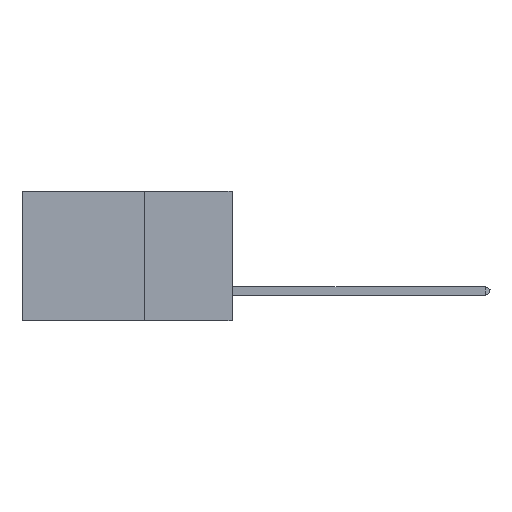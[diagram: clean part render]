
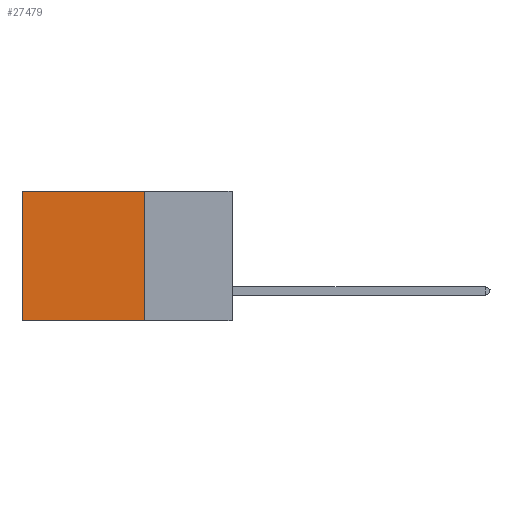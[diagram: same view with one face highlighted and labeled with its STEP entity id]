
A CAD part, left-side view. The second image highlights one B-rep face of the part: STEP entity #27479.
In plain terms, the highlighted planar face has unit normal (-1, 0, 0).
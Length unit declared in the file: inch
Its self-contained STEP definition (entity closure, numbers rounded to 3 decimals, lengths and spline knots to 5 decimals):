
#812 = PLANE ( 'NONE',  #20107 ) ;
#837 = CARTESIAN_POINT ( 'NONE',  ( 0.2875, 0.6, 0. ) ) ;
#2189 = EDGE_CURVE ( 'NONE', #25283, #23253, #4001, .T. ) ;
#4001 = LINE ( 'NONE', #10953, #29038 ) ;
#4308 = ORIENTED_EDGE ( 'NONE', *, *, #27179, .T. ) ;
#5876 = CARTESIAN_POINT ( 'NONE',  ( 0.2875, 0.25, 0. ) ) ;
#6701 = VERTEX_POINT ( 'NONE', #24163 ) ;
#7078 = LINE ( 'NONE', #837, #10500 ) ;
#7468 = EDGE_CURVE ( 'NONE', #6701, #9893, #19962, .T. ) ;
#7688 = VECTOR ( 'NONE', #10622, 39.37008 ) ;
#8294 = ORIENTED_EDGE ( 'NONE', *, *, #2189, .F. ) ;
#8321 = EDGE_CURVE ( 'NONE', #6701, #25283, #19513, .T. ) ;
#8379 = DIRECTION ( 'NONE',  ( 0., 1., 0. ) ) ;
#8865 = ORIENTED_EDGE ( 'NONE', *, *, #7468, .T. ) ;
#9514 = EDGE_LOOP ( 'NONE', ( #4308, #8294, #21635, #8865 ) ) ;
#9893 = VERTEX_POINT ( 'NONE', #20082 ) ;
#10471 = VECTOR ( 'NONE', #8379, 39.37008 ) ;
#10500 = VECTOR ( 'NONE', #17503, 39.37008 ) ;
#10622 = DIRECTION ( 'NONE',  ( 0., 0., -1. ) ) ;
#10794 = DIRECTION ( 'NONE',  ( 0., 0., -1. ) ) ;
#10953 = CARTESIAN_POINT ( 'NONE',  ( 0.2875, 0.25, -0.37 ) ) ;
#14301 = FACE_OUTER_BOUND ( 'NONE', #9514, .T. ) ;
#17503 = DIRECTION ( 'NONE',  ( 0., 0., -1. ) ) ;
#19513 = LINE ( 'NONE', #19745, #7688 ) ;
#19745 = CARTESIAN_POINT ( 'NONE',  ( 0.2875, 0.25, 0. ) ) ;
#19962 = LINE ( 'NONE', #20490, #10471 ) ;
#20082 = CARTESIAN_POINT ( 'NONE',  ( 0.2875, 0.6, 0. ) ) ;
#20107 = AXIS2_PLACEMENT_3D ( 'NONE', #5876, #30510, #10794 ) ;
#20490 = CARTESIAN_POINT ( 'NONE',  ( 0.2875, 0.25, 0. ) ) ;
#21635 = ORIENTED_EDGE ( 'NONE', *, *, #8321, .F. ) ;
#23253 = VERTEX_POINT ( 'NONE', #25130 ) ;
#24163 = CARTESIAN_POINT ( 'NONE',  ( 0.2875, 0.25, 0. ) ) ;
#25130 = CARTESIAN_POINT ( 'NONE',  ( 0.2875, 0.6, -0.37 ) ) ;
#25283 = VERTEX_POINT ( 'NONE', #26386 ) ;
#26386 = CARTESIAN_POINT ( 'NONE',  ( 0.2875, 0.25, -0.37 ) ) ;
#27179 = EDGE_CURVE ( 'NONE', #9893, #23253, #7078, .T. ) ;
#27479 = ADVANCED_FACE ( 'NONE', ( #14301 ), #812, .F. ) ;
#29038 = VECTOR ( 'NONE', #30336, 39.37008 ) ;
#30336 = DIRECTION ( 'NONE',  ( 0., 1., 0. ) ) ;
#30510 = DIRECTION ( 'NONE',  ( 1., 0., 0. ) ) ;
